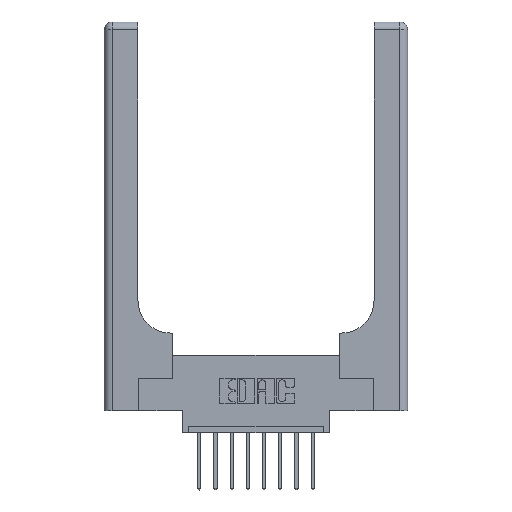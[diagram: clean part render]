
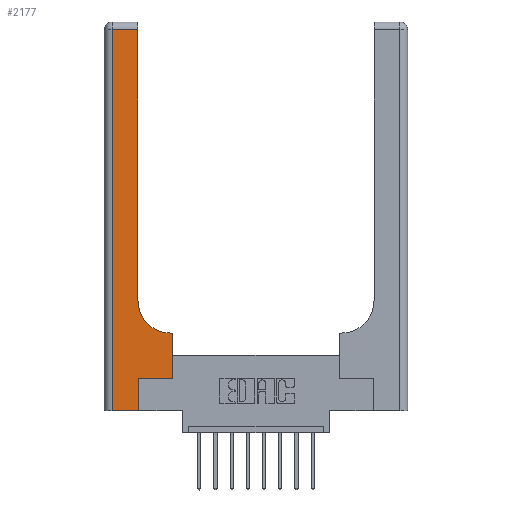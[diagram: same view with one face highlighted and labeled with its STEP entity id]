
A CAD part, top view. The second image highlights one B-rep face of the part: STEP entity #2177.
In plain terms, the highlighted planar face has unit normal (0, 0, 1).
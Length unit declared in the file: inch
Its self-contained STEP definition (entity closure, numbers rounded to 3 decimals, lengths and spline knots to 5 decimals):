
#129 = CARTESIAN_POINT ( 'NONE',  ( 0.26, 2.94, 0.37 ) ) ;
#225 = EDGE_CURVE ( 'NONE', #8393, #6343, #13776, .T. ) ;
#509 = CARTESIAN_POINT ( 'NONE',  ( 0.26, 3., 0.37 ) ) ;
#558 = CARTESIAN_POINT ( 'NONE',  ( 0.06, 0., 0.37 ) ) ;
#826 = EDGE_LOOP ( 'NONE', ( #1569, #4565, #8014, #3853, #7289, #1818, #11434, #7317, #8782 ) ) ;
#1220 = AXIS2_PLACEMENT_3D ( 'NONE', #2430, #5685, #8128 ) ;
#1270 = LINE ( 'NONE', #8627, #3592 ) ;
#1569 = ORIENTED_EDGE ( 'NONE', *, *, #14112, .T. ) ;
#1602 = VERTEX_POINT ( 'NONE', #14232 ) ;
#1699 = VECTOR ( 'NONE', #10681, 39.37008 ) ;
#1713 = CARTESIAN_POINT ( 'NONE',  ( 0.26, 0.6, 0.37 ) ) ;
#1818 = ORIENTED_EDGE ( 'NONE', *, *, #2805, .T. ) ;
#1981 = CARTESIAN_POINT ( 'NONE',  ( 0.51, 0.6, 0.37 ) ) ;
#2036 = AXIS2_PLACEMENT_3D ( 'NONE', #4655, #9229, #14396 ) ;
#2112 = CARTESIAN_POINT ( 'NONE',  ( 0.528, 0.6, 0.37 ) ) ;
#2177 = ADVANCED_FACE ( 'NONE', ( #12670 ), #3401, .F. ) ;
#2430 = CARTESIAN_POINT ( 'NONE',  ( 0., 3., 0.37 ) ) ;
#2805 = EDGE_CURVE ( 'NONE', #11465, #7884, #13197, .T. ) ;
#3401 = PLANE ( 'NONE',  #1220 ) ;
#3441 = VECTOR ( 'NONE', #8630, 39.37008 ) ;
#3592 = VECTOR ( 'NONE', #5022, 39.37008 ) ;
#3853 = ORIENTED_EDGE ( 'NONE', *, *, #5233, .T. ) ;
#3925 = LINE ( 'NONE', #12064, #6787 ) ;
#4151 = LINE ( 'NONE', #6203, #4529 ) ;
#4308 = CARTESIAN_POINT ( 'NONE',  ( 0.06, 2.94, 0.37 ) ) ;
#4529 = VECTOR ( 'NONE', #14297, 39.37008 ) ;
#4565 = ORIENTED_EDGE ( 'NONE', *, *, #11365, .T. ) ;
#4655 = CARTESIAN_POINT ( 'NONE',  ( 0.51, 0.85, 0.37 ) ) ;
#4674 = VECTOR ( 'NONE', #7417, 39.37008 ) ;
#5022 = DIRECTION ( 'NONE',  ( 1., 0., 0. ) ) ;
#5233 = EDGE_CURVE ( 'NONE', #5722, #1602, #1270, .T. ) ;
#5685 = DIRECTION ( 'NONE',  ( 0., 0., -1. ) ) ;
#5722 = VERTEX_POINT ( 'NONE', #558 ) ;
#5854 = LINE ( 'NONE', #10535, #11970 ) ;
#6122 = EDGE_CURVE ( 'NONE', #7884, #14305, #3925, .T. ) ;
#6171 = VECTOR ( 'NONE', #8910, 39.37008 ) ;
#6203 = CARTESIAN_POINT ( 'NONE',  ( 0.265, 0., 0.37 ) ) ;
#6247 = VERTEX_POINT ( 'NONE', #4308 ) ;
#6289 = LINE ( 'NONE', #1713, #4674 ) ;
#6343 = VERTEX_POINT ( 'NONE', #11190 ) ;
#6505 = LINE ( 'NONE', #509, #3441 ) ;
#6787 = VECTOR ( 'NONE', #8547, 39.37008 ) ;
#6939 = CARTESIAN_POINT ( 'NONE',  ( 0.528, 0.25, 0.37 ) ) ;
#7029 = EDGE_CURVE ( 'NONE', #14305, #8393, #6289, .T. ) ;
#7289 = ORIENTED_EDGE ( 'NONE', *, *, #14624, .T. ) ;
#7317 = ORIENTED_EDGE ( 'NONE', *, *, #7029, .T. ) ;
#7417 = DIRECTION ( 'NONE',  ( -1., 0., 0. ) ) ;
#7884 = VERTEX_POINT ( 'NONE', #6939 ) ;
#8014 = ORIENTED_EDGE ( 'NONE', *, *, #14006, .T. ) ;
#8128 = DIRECTION ( 'NONE',  ( -1., 0., 0. ) ) ;
#8393 = VERTEX_POINT ( 'NONE', #1981 ) ;
#8521 = CARTESIAN_POINT ( 'NONE',  ( 0.265, 0.25, 0.37 ) ) ;
#8547 = DIRECTION ( 'NONE',  ( 0., 1., 0. ) ) ;
#8627 = CARTESIAN_POINT ( 'NONE',  ( 0., 0., 0.37 ) ) ;
#8630 = DIRECTION ( 'NONE',  ( 0., 1., 0. ) ) ;
#8782 = ORIENTED_EDGE ( 'NONE', *, *, #225, .T. ) ;
#8910 = DIRECTION ( 'NONE',  ( 1., 0., 0. ) ) ;
#9229 = DIRECTION ( 'NONE',  ( 0., 0., -1. ) ) ;
#10009 = CARTESIAN_POINT ( 'NONE',  ( 0.265, 0.25, 0.37 ) ) ;
#10346 = VERTEX_POINT ( 'NONE', #129 ) ;
#10497 = CARTESIAN_POINT ( 'NONE',  ( 0.06, 3., 0.37 ) ) ;
#10535 = CARTESIAN_POINT ( 'NONE',  ( 0., 2.94, 0.37 ) ) ;
#10681 = DIRECTION ( 'NONE',  ( 0., -1., 0. ) ) ;
#11190 = CARTESIAN_POINT ( 'NONE',  ( 0.26, 0.85, 0.37 ) ) ;
#11220 = LINE ( 'NONE', #10497, #1699 ) ;
#11365 = EDGE_CURVE ( 'NONE', #10346, #6247, #5854, .T. ) ;
#11434 = ORIENTED_EDGE ( 'NONE', *, *, #6122, .T. ) ;
#11465 = VERTEX_POINT ( 'NONE', #8521 ) ;
#11970 = VECTOR ( 'NONE', #12775, 39.37008 ) ;
#12064 = CARTESIAN_POINT ( 'NONE',  ( 0.528, 0.25, 0.37 ) ) ;
#12670 = FACE_OUTER_BOUND ( 'NONE', #826, .T. ) ;
#12775 = DIRECTION ( 'NONE',  ( -1., 0., 0. ) ) ;
#13197 = LINE ( 'NONE', #10009, #6171 ) ;
#13776 = CIRCLE ( 'NONE', #2036, 0.25 ) ;
#14006 = EDGE_CURVE ( 'NONE', #6247, #5722, #11220, .T. ) ;
#14112 = EDGE_CURVE ( 'NONE', #6343, #10346, #6505, .T. ) ;
#14232 = CARTESIAN_POINT ( 'NONE',  ( 0.265, 0., 0.37 ) ) ;
#14297 = DIRECTION ( 'NONE',  ( 0., 1., 0. ) ) ;
#14305 = VERTEX_POINT ( 'NONE', #2112 ) ;
#14396 = DIRECTION ( 'NONE',  ( 1., 0., 0. ) ) ;
#14624 = EDGE_CURVE ( 'NONE', #1602, #11465, #4151, .T. ) ;
